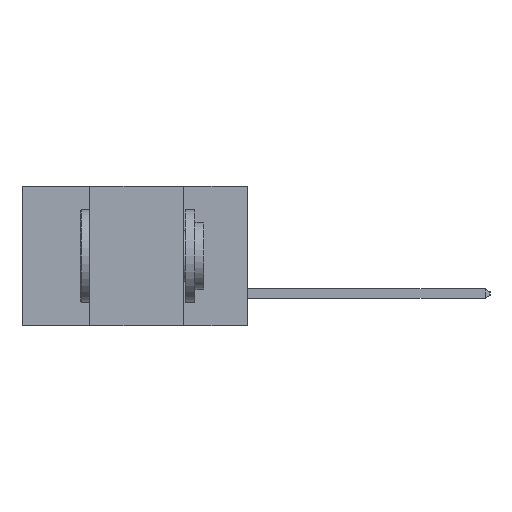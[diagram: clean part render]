
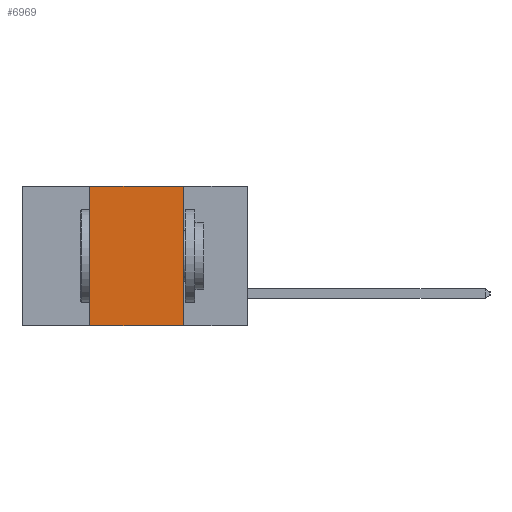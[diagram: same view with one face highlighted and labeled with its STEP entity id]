
A CAD part, left-side view. The second image highlights one B-rep face of the part: STEP entity #6969.
In plain terms, the highlighted planar face has unit normal (-1, 0, 0).
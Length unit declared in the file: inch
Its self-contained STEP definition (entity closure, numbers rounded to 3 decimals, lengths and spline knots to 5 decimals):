
#128 = CARTESIAN_POINT ( 'NONE',  ( 0., 0.42, 0. ) ) ;
#714 = CARTESIAN_POINT ( 'NONE',  ( 0., 0.17, 0. ) ) ;
#847 = ORIENTED_EDGE ( 'NONE', *, *, #13581, .F. ) ;
#1299 = FACE_OUTER_BOUND ( 'NONE', #2215, .T. ) ;
#1612 = CARTESIAN_POINT ( 'NONE',  ( 0., 0.42, -0.37 ) ) ;
#2215 = EDGE_LOOP ( 'NONE', ( #12569, #4833, #847, #14103 ) ) ;
#2546 = CARTESIAN_POINT ( 'NONE',  ( 0., 0.6, 0. ) ) ;
#2987 = EDGE_CURVE ( 'NONE', #3341, #3225, #9970, .T. ) ;
#3225 = VERTEX_POINT ( 'NONE', #3335 ) ;
#3335 = CARTESIAN_POINT ( 'NONE',  ( 0., 0.17, -0.37 ) ) ;
#3341 = VERTEX_POINT ( 'NONE', #1612 ) ;
#4833 = ORIENTED_EDGE ( 'NONE', *, *, #9470, .F. ) ;
#5112 = DIRECTION ( 'NONE',  ( 1., 0., 0. ) ) ;
#5604 = VECTOR ( 'NONE', #14213, 39.37008 ) ;
#5710 = LINE ( 'NONE', #5919, #6488 ) ;
#5825 = AXIS2_PLACEMENT_3D ( 'NONE', #2546, #5112, #13242 ) ;
#5919 = CARTESIAN_POINT ( 'NONE',  ( 0., 0.42, -0.37 ) ) ;
#6002 = LINE ( 'NONE', #15308, #5604 ) ;
#6488 = VECTOR ( 'NONE', #13934, 39.37008 ) ;
#6637 = DIRECTION ( 'NONE',  ( 0., -1., 0. ) ) ;
#6683 = VERTEX_POINT ( 'NONE', #714 ) ;
#6792 = EDGE_CURVE ( 'NONE', #6683, #3225, #7372, .T. ) ;
#6890 = VECTOR ( 'NONE', #6637, 39.37008 ) ;
#6969 = ADVANCED_FACE ( 'NONE', ( #1299 ), #8661, .F. ) ;
#7076 = CARTESIAN_POINT ( 'NONE',  ( 0., 0.6, -0.37 ) ) ;
#7179 = DIRECTION ( 'NONE',  ( 0., 0., -1. ) ) ;
#7372 = LINE ( 'NONE', #8360, #13118 ) ;
#8360 = CARTESIAN_POINT ( 'NONE',  ( 0., 0.17, -0.37 ) ) ;
#8661 = PLANE ( 'NONE',  #5825 ) ;
#9470 = EDGE_CURVE ( 'NONE', #9963, #6683, #6002, .T. ) ;
#9963 = VERTEX_POINT ( 'NONE', #128 ) ;
#9970 = LINE ( 'NONE', #7076, #6890 ) ;
#12569 = ORIENTED_EDGE ( 'NONE', *, *, #6792, .F. ) ;
#13118 = VECTOR ( 'NONE', #7179, 39.37008 ) ;
#13242 = DIRECTION ( 'NONE',  ( 0., 0., -1. ) ) ;
#13581 = EDGE_CURVE ( 'NONE', #3341, #9963, #5710, .T. ) ;
#13934 = DIRECTION ( 'NONE',  ( 0., 0., 1. ) ) ;
#14103 = ORIENTED_EDGE ( 'NONE', *, *, #2987, .T. ) ;
#14213 = DIRECTION ( 'NONE',  ( 0., -1., 0. ) ) ;
#15308 = CARTESIAN_POINT ( 'NONE',  ( 0., 0.6, 0. ) ) ;
